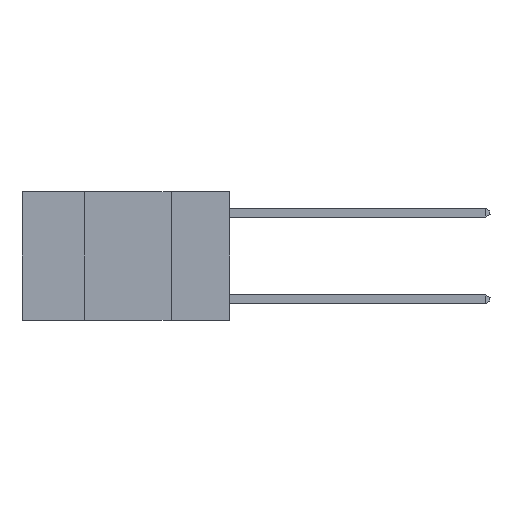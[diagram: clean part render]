
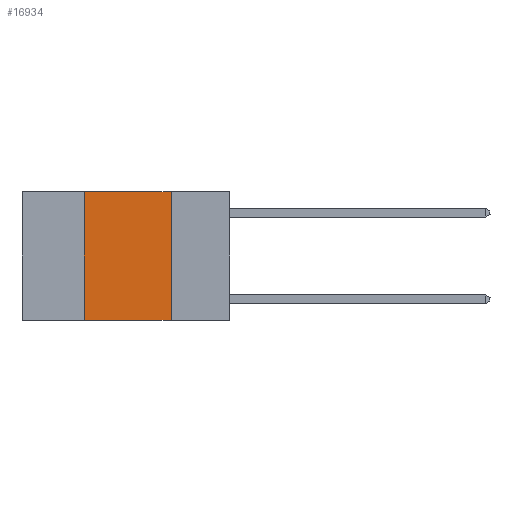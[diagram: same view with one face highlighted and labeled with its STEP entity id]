
A CAD part, left-side view. The second image highlights one B-rep face of the part: STEP entity #16934.
In plain terms, the highlighted planar face has unit normal (-1, 0, 0).
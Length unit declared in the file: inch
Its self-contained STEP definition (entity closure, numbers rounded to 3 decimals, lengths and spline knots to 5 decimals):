
#68 = DIRECTION ( 'NONE',  ( 0., -1., 0. ) ) ;
#231 = PLANE ( 'NONE',  #5822 ) ;
#1279 = EDGE_LOOP ( 'NONE', ( #9350, #16316, #12494, #15817 ) ) ;
#1595 = LINE ( 'NONE', #14643, #18123 ) ;
#2515 = VERTEX_POINT ( 'NONE', #5313 ) ;
#2910 = EDGE_CURVE ( 'NONE', #9805, #2515, #8046, .T. ) ;
#2946 = DIRECTION ( 'NONE',  ( 0., 0., -1. ) ) ;
#3744 = CARTESIAN_POINT ( 'NONE',  ( 0., 0.42, -0.37 ) ) ;
#3922 = VERTEX_POINT ( 'NONE', #19064 ) ;
#4386 = EDGE_CURVE ( 'NONE', #9805, #12258, #5677, .T. ) ;
#4743 = CARTESIAN_POINT ( 'NONE',  ( 0., 0.6, 0. ) ) ;
#5313 = CARTESIAN_POINT ( 'NONE',  ( 0., 0.42, 0. ) ) ;
#5677 = LINE ( 'NONE', #14644, #12211 ) ;
#5822 = AXIS2_PLACEMENT_3D ( 'NONE', #4743, #14814, #11976 ) ;
#5920 = CARTESIAN_POINT ( 'NONE',  ( 0., 0.17, -0.37 ) ) ;
#8046 = LINE ( 'NONE', #13976, #17622 ) ;
#8469 = VECTOR ( 'NONE', #16998, 39.37008 ) ;
#9350 = ORIENTED_EDGE ( 'NONE', *, *, #9984, .F. ) ;
#9630 = EDGE_CURVE ( 'NONE', #2515, #3922, #10940, .T. ) ;
#9805 = VERTEX_POINT ( 'NONE', #3744 ) ;
#9984 = EDGE_CURVE ( 'NONE', #3922, #12258, #1595, .T. ) ;
#10940 = LINE ( 'NONE', #14064, #8469 ) ;
#11976 = DIRECTION ( 'NONE',  ( 0., 0., -1. ) ) ;
#12211 = VECTOR ( 'NONE', #68, 39.37008 ) ;
#12258 = VERTEX_POINT ( 'NONE', #5920 ) ;
#12494 = ORIENTED_EDGE ( 'NONE', *, *, #2910, .F. ) ;
#13976 = CARTESIAN_POINT ( 'NONE',  ( 0., 0.42, 0. ) ) ;
#14064 = CARTESIAN_POINT ( 'NONE',  ( 0., 0.6, 0. ) ) ;
#14643 = CARTESIAN_POINT ( 'NONE',  ( 0., 0.17, 0. ) ) ;
#14644 = CARTESIAN_POINT ( 'NONE',  ( 0., 0.6, -0.37 ) ) ;
#14814 = DIRECTION ( 'NONE',  ( 1., 0., 0. ) ) ;
#15817 = ORIENTED_EDGE ( 'NONE', *, *, #4386, .T. ) ;
#16316 = ORIENTED_EDGE ( 'NONE', *, *, #9630, .F. ) ;
#16934 = ADVANCED_FACE ( 'NONE', ( #17824 ), #231, .F. ) ;
#16998 = DIRECTION ( 'NONE',  ( 0., -1., 0. ) ) ;
#17622 = VECTOR ( 'NONE', #18567, 39.37008 ) ;
#17824 = FACE_OUTER_BOUND ( 'NONE', #1279, .T. ) ;
#18123 = VECTOR ( 'NONE', #2946, 39.37008 ) ;
#18567 = DIRECTION ( 'NONE',  ( 0., 0., 1. ) ) ;
#19064 = CARTESIAN_POINT ( 'NONE',  ( 0., 0.17, 0. ) ) ;
